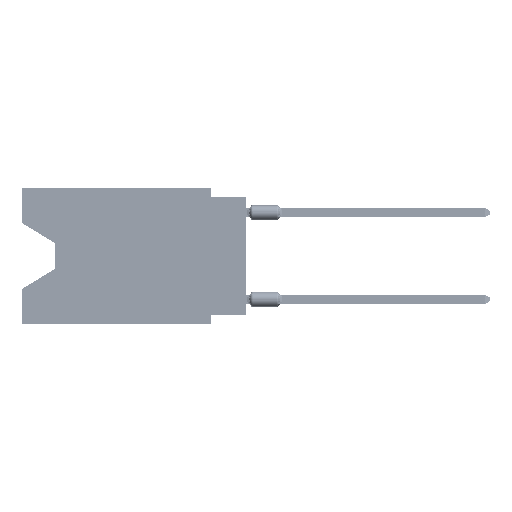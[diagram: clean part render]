
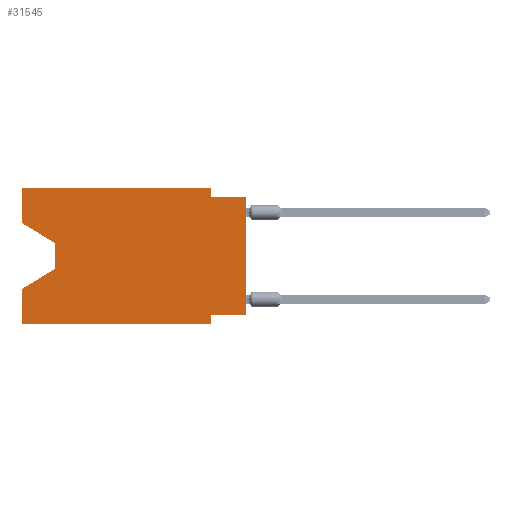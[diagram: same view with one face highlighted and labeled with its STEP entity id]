
A CAD part, left-side view. The second image highlights one B-rep face of the part: STEP entity #31545.
In plain terms, the highlighted planar face has unit normal (-1, 0, 0).
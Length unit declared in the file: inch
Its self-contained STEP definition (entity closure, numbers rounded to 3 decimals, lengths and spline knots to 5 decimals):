
#1337 = EDGE_CURVE ( 'NONE', #9446, #45459, #36290, .T. ) ;
#1451 = CARTESIAN_POINT ( 'NONE',  ( 0., 0.645, 0. ) ) ;
#2291 = EDGE_CURVE ( 'NONE', #67563, #45244, #64784, .T. ) ;
#3063 = VECTOR ( 'NONE', #48431, 39.37008 ) ;
#4239 = CARTESIAN_POINT ( 'NONE',  ( 0., 0.645, 0. ) ) ;
#5298 = CARTESIAN_POINT ( 'NONE',  ( 0., 0.645, 0. ) ) ;
#5526 = ORIENTED_EDGE ( 'NONE', *, *, #37434, .T. ) ;
#5946 = CARTESIAN_POINT ( 'NONE',  ( 0., 0.55, -0.232 ) ) ;
#6111 = DIRECTION ( 'NONE',  ( 0., 0., 1. ) ) ;
#9268 = EDGE_CURVE ( 'NONE', #56305, #18282, #46215, .T. ) ;
#9446 = VERTEX_POINT ( 'NONE', #48233 ) ;
#10528 = CARTESIAN_POINT ( 'NONE',  ( 0., 0., -0.365 ) ) ;
#10708 = CARTESIAN_POINT ( 'NONE',  ( 0., 0.645, 0. ) ) ;
#11940 = LINE ( 'NONE', #10708, #37278 ) ;
#12346 = DIRECTION ( 'NONE',  ( 0., -1., 0. ) ) ;
#12438 = VERTEX_POINT ( 'NONE', #26953 ) ;
#12600 = LINE ( 'NONE', #37823, #52484 ) ;
#13107 = ORIENTED_EDGE ( 'NONE', *, *, #2291, .F. ) ;
#13402 = DIRECTION ( 'NONE',  ( 1., 0., 0. ) ) ;
#14180 = DIRECTION ( 'NONE',  ( 0., 1., 0. ) ) ;
#14372 = CARTESIAN_POINT ( 'NONE',  ( 0., 0.1, -0.39 ) ) ;
#14519 = ORIENTED_EDGE ( 'NONE', *, *, #74503, .T. ) ;
#17406 = ORIENTED_EDGE ( 'NONE', *, *, #19707, .T. ) ;
#17830 = CARTESIAN_POINT ( 'NONE',  ( 0., 0.1, -0.365 ) ) ;
#18282 = VERTEX_POINT ( 'NONE', #27601 ) ;
#18309 = ORIENTED_EDGE ( 'NONE', *, *, #1337, .F. ) ;
#18650 = ORIENTED_EDGE ( 'NONE', *, *, #9268, .F. ) ;
#19707 = EDGE_CURVE ( 'NONE', #27101, #22929, #74671, .T. ) ;
#21425 = EDGE_CURVE ( 'NONE', #67406, #62952, #12600, .T. ) ;
#22205 = CARTESIAN_POINT ( 'NONE',  ( 0., 0.1, 0. ) ) ;
#22929 = VERTEX_POINT ( 'NONE', #45152 ) ;
#23200 = CARTESIAN_POINT ( 'NONE',  ( 0., 0.55, -0.232 ) ) ;
#26114 = EDGE_CURVE ( 'NONE', #27101, #56305, #40217, .T. ) ;
#26953 = CARTESIAN_POINT ( 'NONE',  ( 0., 0.645, -0.39 ) ) ;
#27101 = VERTEX_POINT ( 'NONE', #10528 ) ;
#27509 = ORIENTED_EDGE ( 'NONE', *, *, #28929, .T. ) ;
#27601 = CARTESIAN_POINT ( 'NONE',  ( 0., 0.1, -0.39 ) ) ;
#28649 = AXIS2_PLACEMENT_3D ( 'NONE', #47059, #13402, #51419 ) ;
#28766 = LINE ( 'NONE', #35801, #73284 ) ;
#28929 = EDGE_CURVE ( 'NONE', #12438, #18282, #32725, .T. ) ;
#29417 = LINE ( 'NONE', #23200, #3063 ) ;
#29845 = ORIENTED_EDGE ( 'NONE', *, *, #51214, .F. ) ;
#31545 = ADVANCED_FACE ( 'NONE', ( #34234 ), #78407, .F. ) ;
#32725 = LINE ( 'NONE', #40555, #77165 ) ;
#34234 = FACE_OUTER_BOUND ( 'NONE', #77466, .T. ) ;
#35801 = CARTESIAN_POINT ( 'NONE',  ( 0., 0., -0.025 ) ) ;
#36290 = LINE ( 'NONE', #5298, #52855 ) ;
#37278 = VECTOR ( 'NONE', #12346, 39.37008 ) ;
#37346 = ORIENTED_EDGE ( 'NONE', *, *, #21425, .T. ) ;
#37434 = EDGE_CURVE ( 'NONE', #62952, #46074, #29417, .T. ) ;
#37823 = CARTESIAN_POINT ( 'NONE',  ( 0., 0.55, -0.158 ) ) ;
#37966 = ORIENTED_EDGE ( 'NONE', *, *, #43460, .F. ) ;
#39617 = CARTESIAN_POINT ( 'NONE',  ( 0., 0.1, -0.025 ) ) ;
#40217 = LINE ( 'NONE', #44805, #67421 ) ;
#40555 = CARTESIAN_POINT ( 'NONE',  ( 0., 0.645, -0.39 ) ) ;
#43460 = EDGE_CURVE ( 'NONE', #12438, #46074, #54633, .T. ) ;
#44805 = CARTESIAN_POINT ( 'NONE',  ( 0., 0., -0.365 ) ) ;
#45152 = CARTESIAN_POINT ( 'NONE',  ( 0., 0., -0.025 ) ) ;
#45244 = VERTEX_POINT ( 'NONE', #39617 ) ;
#45459 = VERTEX_POINT ( 'NONE', #1451 ) ;
#46074 = VERTEX_POINT ( 'NONE', #47600 ) ;
#46215 = LINE ( 'NONE', #14372, #48199 ) ;
#46351 = DIRECTION ( 'NONE',  ( 0., -1., 0. ) ) ;
#47039 = CARTESIAN_POINT ( 'NONE',  ( 0., 0.55, -0.158 ) ) ;
#47059 = CARTESIAN_POINT ( 'NONE',  ( 0., 0.645, 0. ) ) ;
#47600 = CARTESIAN_POINT ( 'NONE',  ( 0., 0.645, -0.28975 ) ) ;
#48199 = VECTOR ( 'NONE', #52389, 39.37008 ) ;
#48233 = CARTESIAN_POINT ( 'NONE',  ( 0., 0.645, -0.10025 ) ) ;
#48431 = DIRECTION ( 'NONE',  ( 0., 0.855, -0.519 ) ) ;
#48725 = CARTESIAN_POINT ( 'NONE',  ( 0., 0.645, -0.10025 ) ) ;
#51033 = DIRECTION ( 'NONE',  ( 0., 0., -1. ) ) ;
#51214 = EDGE_CURVE ( 'NONE', #45459, #67563, #11940, .T. ) ;
#51419 = DIRECTION ( 'NONE',  ( 0., 0., -1. ) ) ;
#51988 = DIRECTION ( 'NONE',  ( 0., 0., -1. ) ) ;
#52389 = DIRECTION ( 'NONE',  ( 0., 0., -1. ) ) ;
#52484 = VECTOR ( 'NONE', #51033, 39.37008 ) ;
#52855 = VECTOR ( 'NONE', #6111, 39.37008 ) ;
#54633 = LINE ( 'NONE', #4239, #75784 ) ;
#54906 = DIRECTION ( 'NONE',  ( 0., -0.855, -0.519 ) ) ;
#55267 = DIRECTION ( 'NONE',  ( 0., 0., 1. ) ) ;
#56305 = VERTEX_POINT ( 'NONE', #17830 ) ;
#57191 = VECTOR ( 'NONE', #54906, 39.37008 ) ;
#57405 = EDGE_CURVE ( 'NONE', #45244, #22929, #28766, .T. ) ;
#59808 = CARTESIAN_POINT ( 'NONE',  ( 0., 0.1, 0. ) ) ;
#62952 = VERTEX_POINT ( 'NONE', #5946 ) ;
#64784 = LINE ( 'NONE', #59808, #67184 ) ;
#66555 = VECTOR ( 'NONE', #55267, 39.37008 ) ;
#67175 = DIRECTION ( 'NONE',  ( 0., -1., 0. ) ) ;
#67184 = VECTOR ( 'NONE', #51988, 39.37008 ) ;
#67406 = VERTEX_POINT ( 'NONE', #47039 ) ;
#67421 = VECTOR ( 'NONE', #14180, 39.37008 ) ;
#67563 = VERTEX_POINT ( 'NONE', #22205 ) ;
#73284 = VECTOR ( 'NONE', #67175, 39.37008 ) ;
#73614 = DIRECTION ( 'NONE',  ( 0., 0., 1. ) ) ;
#74503 = EDGE_CURVE ( 'NONE', #9446, #67406, #80516, .T. ) ;
#74671 = LINE ( 'NONE', #80467, #66555 ) ;
#75439 = ORIENTED_EDGE ( 'NONE', *, *, #26114, .F. ) ;
#75784 = VECTOR ( 'NONE', #73614, 39.37008 ) ;
#77165 = VECTOR ( 'NONE', #46351, 39.37008 ) ;
#77466 = EDGE_LOOP ( 'NONE', ( #14519, #37346, #5526, #37966, #27509, #18650, #75439, #17406, #79946, #13107, #29845, #18309 ) ) ;
#78407 = PLANE ( 'NONE',  #28649 ) ;
#79946 = ORIENTED_EDGE ( 'NONE', *, *, #57405, .F. ) ;
#80467 = CARTESIAN_POINT ( 'NONE',  ( 0., 0., 0. ) ) ;
#80516 = LINE ( 'NONE', #48725, #57191 ) ;
